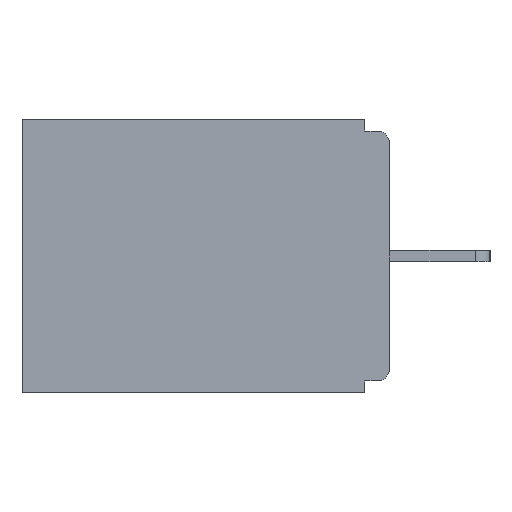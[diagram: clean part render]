
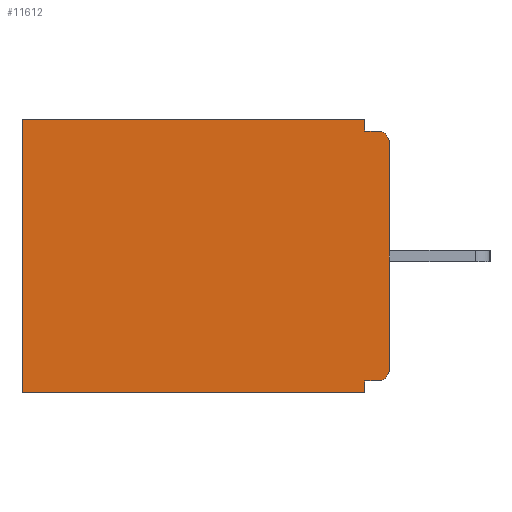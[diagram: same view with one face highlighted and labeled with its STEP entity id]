
A CAD part, left-side view. The second image highlights one B-rep face of the part: STEP entity #11612.
In plain terms, the highlighted planar face has unit normal (-1, 0, 0).
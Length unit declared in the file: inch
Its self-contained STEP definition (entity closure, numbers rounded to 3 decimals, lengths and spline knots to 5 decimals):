
#273 = CARTESIAN_POINT ( 'NONE',  ( 0.298, 0., -0.313 ) ) ;
#366 = VECTOR ( 'NONE', #24956, 39.37008 ) ;
#711 = CARTESIAN_POINT ( 'NONE',  ( 0.298, 0.031, -0.343 ) ) ;
#1310 = EDGE_CURVE ( 'NONE', #5538, #13478, #20892, .T. ) ;
#1454 = ORIENTED_EDGE ( 'NONE', *, *, #21887, .T. ) ;
#1932 = CARTESIAN_POINT ( 'NONE',  ( 0.298, 0.031, -0.015 ) ) ;
#2271 = VERTEX_POINT ( 'NONE', #21585 ) ;
#2885 = DIRECTION ( 'NONE',  ( -1., 0., 0. ) ) ;
#3706 = ORIENTED_EDGE ( 'NONE', *, *, #7053, .F. ) ;
#3779 = LINE ( 'NONE', #16597, #23763 ) ;
#3910 = ORIENTED_EDGE ( 'NONE', *, *, #24555, .F. ) ;
#3947 = VECTOR ( 'NONE', #22187, 39.37008 ) ;
#4124 = EDGE_CURVE ( 'NONE', #22712, #12217, #3779, .T. ) ;
#4852 = CARTESIAN_POINT ( 'NONE',  ( 0.298, 0.015, -0.328 ) ) ;
#4928 = EDGE_CURVE ( 'NONE', #6014, #19502, #11404, .T. ) ;
#5216 = VERTEX_POINT ( 'NONE', #24384 ) ;
#5273 = EDGE_CURVE ( 'NONE', #12217, #7575, #13792, .T. ) ;
#5307 = DIRECTION ( 'NONE',  ( 0., 0., -1. ) ) ;
#5518 = LINE ( 'NONE', #22146, #23629 ) ;
#5538 = VERTEX_POINT ( 'NONE', #4852 ) ;
#5709 = CARTESIAN_POINT ( 'NONE',  ( 0.298, 0.031, -0.328 ) ) ;
#6014 = VERTEX_POINT ( 'NONE', #711 ) ;
#6222 = VECTOR ( 'NONE', #11651, 39.37008 ) ;
#6803 = DIRECTION ( 'NONE',  ( 0., 1., 0. ) ) ;
#7053 = EDGE_CURVE ( 'NONE', #5216, #13478, #7968, .T. ) ;
#7285 = CARTESIAN_POINT ( 'NONE',  ( 0.298, 0.031, -0.343 ) ) ;
#7575 = VERTEX_POINT ( 'NONE', #10368 ) ;
#7828 = ORIENTED_EDGE ( 'NONE', *, *, #4928, .F. ) ;
#7968 = LINE ( 'NONE', #20109, #3947 ) ;
#8194 = CARTESIAN_POINT ( 'NONE',  ( 0.298, 0.46, -0.343 ) ) ;
#8416 = ORIENTED_EDGE ( 'NONE', *, *, #18483, .T. ) ;
#8659 = VECTOR ( 'NONE', #23521, 39.37008 ) ;
#8696 = ORIENTED_EDGE ( 'NONE', *, *, #1310, .T. ) ;
#8704 = LINE ( 'NONE', #9572, #23448 ) ;
#8726 = AXIS2_PLACEMENT_3D ( 'NONE', #10905, #24334, #12821 ) ;
#9572 = CARTESIAN_POINT ( 'NONE',  ( 0.298, 0., -0.328 ) ) ;
#10368 = CARTESIAN_POINT ( 'NONE',  ( 0.298, 0.015, -0.015 ) ) ;
#10905 = CARTESIAN_POINT ( 'NONE',  ( 0.298, 0., 0. ) ) ;
#11404 = LINE ( 'NONE', #18590, #6222 ) ;
#11612 = ADVANCED_FACE ( 'NONE', ( #20740 ), #18526, .F. ) ;
#11651 = DIRECTION ( 'NONE',  ( 0., 1., 0. ) ) ;
#12146 = ORIENTED_EDGE ( 'NONE', *, *, #24461, .F. ) ;
#12217 = VERTEX_POINT ( 'NONE', #1932 ) ;
#12324 = ORIENTED_EDGE ( 'NONE', *, *, #12782, .T. ) ;
#12782 = EDGE_CURVE ( 'NONE', #2271, #19502, #16021, .T. ) ;
#12821 = DIRECTION ( 'NONE',  ( 0., 0., -1. ) ) ;
#13478 = VERTEX_POINT ( 'NONE', #273 ) ;
#13792 = LINE ( 'NONE', #24024, #8659 ) ;
#14561 = CARTESIAN_POINT ( 'NONE',  ( 0.298, 0.015, -0.03 ) ) ;
#15654 = VECTOR ( 'NONE', #5307, 39.37008 ) ;
#16021 = LINE ( 'NONE', #23040, #366 ) ;
#16239 = ORIENTED_EDGE ( 'NONE', *, *, #4124, .F. ) ;
#16272 = LINE ( 'NONE', #7285, #15654 ) ;
#16528 = DIRECTION ( 'NONE',  ( 0., 0., -1. ) ) ;
#16597 = CARTESIAN_POINT ( 'NONE',  ( 0.298, 0.031, -0.343 ) ) ;
#16620 = VERTEX_POINT ( 'NONE', #5709 ) ;
#18306 = ORIENTED_EDGE ( 'NONE', *, *, #5273, .F. ) ;
#18483 = EDGE_CURVE ( 'NONE', #5216, #7575, #19371, .T. ) ;
#18526 = PLANE ( 'NONE',  #8726 ) ;
#18590 = CARTESIAN_POINT ( 'NONE',  ( 0.298, 0., -0.343 ) ) ;
#19371 = CIRCLE ( 'NONE', #24681, 0.015 ) ;
#19502 = VERTEX_POINT ( 'NONE', #8194 ) ;
#19746 = EDGE_LOOP ( 'NONE', ( #8416, #18306, #16239, #1454, #12324, #7828, #12146, #3910, #8696, #3706 ) ) ;
#20109 = CARTESIAN_POINT ( 'NONE',  ( 0.298, 0., 0. ) ) ;
#20740 = FACE_OUTER_BOUND ( 'NONE', #19746, .T. ) ;
#20892 = CIRCLE ( 'NONE', #23456, 0.015 ) ;
#21129 = DIRECTION ( 'NONE',  ( 0., 1., 0. ) ) ;
#21585 = CARTESIAN_POINT ( 'NONE',  ( 0.298, 0.46, 0. ) ) ;
#21887 = EDGE_CURVE ( 'NONE', #22712, #2271, #5518, .T. ) ;
#21932 = DIRECTION ( 'NONE',  ( 0., 0., -1. ) ) ;
#22146 = CARTESIAN_POINT ( 'NONE',  ( 0.298, 0., 0. ) ) ;
#22155 = DIRECTION ( 'NONE',  ( -1., 0., 0. ) ) ;
#22187 = DIRECTION ( 'NONE',  ( 0., 0., -1. ) ) ;
#22712 = VERTEX_POINT ( 'NONE', #22780 ) ;
#22776 = DIRECTION ( 'NONE',  ( 0., 0., -1. ) ) ;
#22780 = CARTESIAN_POINT ( 'NONE',  ( 0.298, 0.031, 0. ) ) ;
#23040 = CARTESIAN_POINT ( 'NONE',  ( 0.298, 0.46, 0. ) ) ;
#23448 = VECTOR ( 'NONE', #21129, 39.37008 ) ;
#23456 = AXIS2_PLACEMENT_3D ( 'NONE', #23716, #22155, #22776 ) ;
#23521 = DIRECTION ( 'NONE',  ( 0., -1., 0. ) ) ;
#23629 = VECTOR ( 'NONE', #6803, 39.37008 ) ;
#23716 = CARTESIAN_POINT ( 'NONE',  ( 0.298, 0.015, -0.313 ) ) ;
#23763 = VECTOR ( 'NONE', #21932, 39.37008 ) ;
#24024 = CARTESIAN_POINT ( 'NONE',  ( 0.298, 0., -0.015 ) ) ;
#24334 = DIRECTION ( 'NONE',  ( 1., 0., 0. ) ) ;
#24384 = CARTESIAN_POINT ( 'NONE',  ( 0.298, 0., -0.03 ) ) ;
#24461 = EDGE_CURVE ( 'NONE', #16620, #6014, #16272, .T. ) ;
#24555 = EDGE_CURVE ( 'NONE', #5538, #16620, #8704, .T. ) ;
#24681 = AXIS2_PLACEMENT_3D ( 'NONE', #14561, #2885, #16528 ) ;
#24956 = DIRECTION ( 'NONE',  ( 0., 0., -1. ) ) ;
